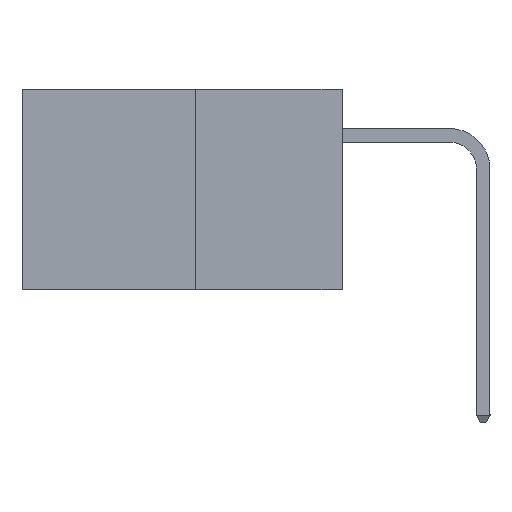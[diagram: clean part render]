
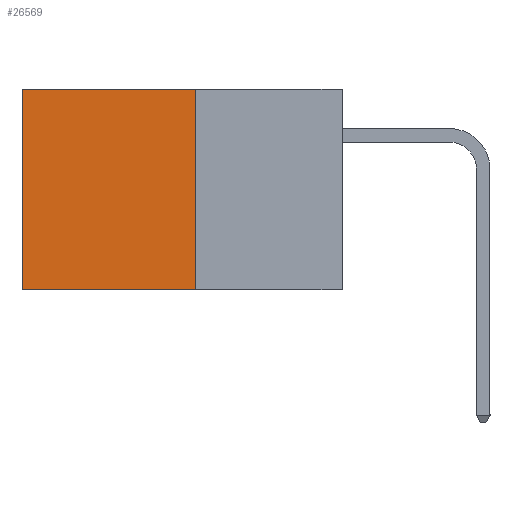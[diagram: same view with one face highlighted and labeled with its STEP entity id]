
A CAD part, left-side view. The second image highlights one B-rep face of the part: STEP entity #26569.
In plain terms, the highlighted planar face has unit normal (-1, 0, 0).
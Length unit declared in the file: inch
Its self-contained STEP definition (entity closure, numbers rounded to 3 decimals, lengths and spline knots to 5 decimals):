
#1398 = CARTESIAN_POINT ( 'NONE',  ( 0.277, 0.27, -0.37 ) ) ;
#1733 = ORIENTED_EDGE ( 'NONE', *, *, #10627, .T. ) ;
#2956 = LINE ( 'NONE', #12910, #13556 ) ;
#3882 = DIRECTION ( 'NONE',  ( 0., 0., -1. ) ) ;
#4600 = VECTOR ( 'NONE', #27260, 39.37008 ) ;
#4740 = DIRECTION ( 'NONE',  ( 0., 0., -1. ) ) ;
#5621 = CARTESIAN_POINT ( 'NONE',  ( 0.277, 0.27, 0. ) ) ;
#6590 = VERTEX_POINT ( 'NONE', #12432 ) ;
#6741 = EDGE_LOOP ( 'NONE', ( #30784, #17904, #15793, #1733 ) ) ;
#8573 = FACE_OUTER_BOUND ( 'NONE', #6741, .T. ) ;
#8611 = VECTOR ( 'NONE', #4740, 39.37008 ) ;
#10627 = EDGE_CURVE ( 'NONE', #6590, #24550, #23796, .T. ) ;
#11528 = AXIS2_PLACEMENT_3D ( 'NONE', #1398, #18295, #3882 ) ;
#12432 = CARTESIAN_POINT ( 'NONE',  ( 0.277, 0.27, 0. ) ) ;
#12910 = CARTESIAN_POINT ( 'NONE',  ( 0.277, 0.27, -0.37 ) ) ;
#13556 = VECTOR ( 'NONE', #22487, 39.37008 ) ;
#14609 = VECTOR ( 'NONE', #21019, 39.37008 ) ;
#15793 = ORIENTED_EDGE ( 'NONE', *, *, #18896, .F. ) ;
#16291 = EDGE_CURVE ( 'NONE', #28872, #20510, #2956, .T. ) ;
#17825 = EDGE_CURVE ( 'NONE', #24550, #20510, #21439, .T. ) ;
#17904 = ORIENTED_EDGE ( 'NONE', *, *, #16291, .F. ) ;
#18295 = DIRECTION ( 'NONE',  ( 1., 0., 0. ) ) ;
#18896 = EDGE_CURVE ( 'NONE', #6590, #28872, #28081, .T. ) ;
#19067 = CARTESIAN_POINT ( 'NONE',  ( 0.277, 0.59, -0.37 ) ) ;
#19291 = CARTESIAN_POINT ( 'NONE',  ( 0.277, 0.27, -0.37 ) ) ;
#20510 = VERTEX_POINT ( 'NONE', #24192 ) ;
#20627 = PLANE ( 'NONE',  #11528 ) ;
#21019 = DIRECTION ( 'NONE',  ( 0., 0., -1. ) ) ;
#21439 = LINE ( 'NONE', #19067, #8611 ) ;
#22487 = DIRECTION ( 'NONE',  ( 0., 1., 0. ) ) ;
#23796 = LINE ( 'NONE', #5621, #4600 ) ;
#24192 = CARTESIAN_POINT ( 'NONE',  ( 0.277, 0.59, -0.37 ) ) ;
#24550 = VERTEX_POINT ( 'NONE', #29482 ) ;
#26569 = ADVANCED_FACE ( 'NONE', ( #8573 ), #20627, .F. ) ;
#27260 = DIRECTION ( 'NONE',  ( 0., 1., 0. ) ) ;
#28081 = LINE ( 'NONE', #28108, #14609 ) ;
#28108 = CARTESIAN_POINT ( 'NONE',  ( 0.277, 0.27, -0.37 ) ) ;
#28872 = VERTEX_POINT ( 'NONE', #19291 ) ;
#29482 = CARTESIAN_POINT ( 'NONE',  ( 0.277, 0.59, 0. ) ) ;
#30784 = ORIENTED_EDGE ( 'NONE', *, *, #17825, .T. ) ;
